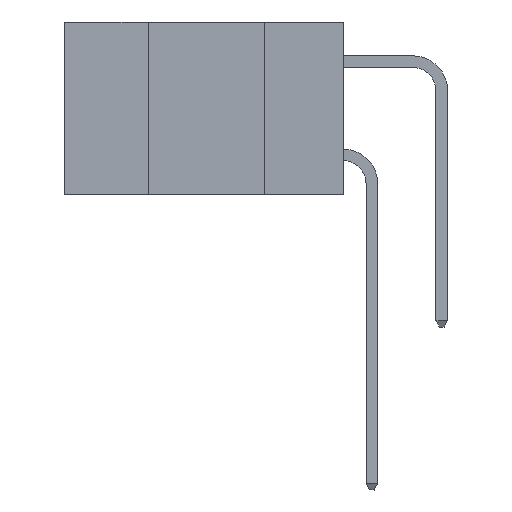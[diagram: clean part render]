
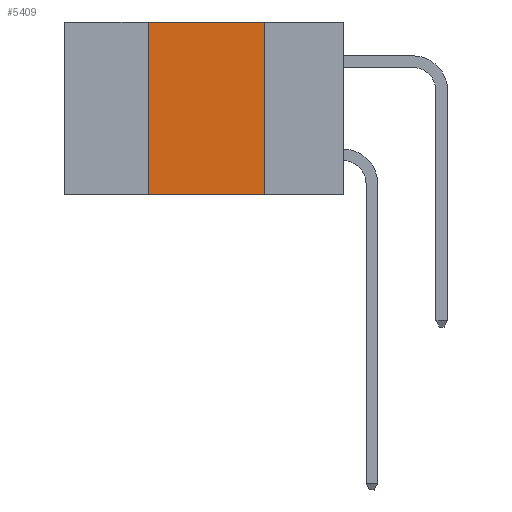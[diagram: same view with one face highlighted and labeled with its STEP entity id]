
A CAD part, left-side view. The second image highlights one B-rep face of the part: STEP entity #5409.
In plain terms, the highlighted planar face has unit normal (-1, 0, 0).
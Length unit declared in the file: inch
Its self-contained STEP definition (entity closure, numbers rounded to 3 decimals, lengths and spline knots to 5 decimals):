
#518 = LINE ( 'NONE', #1410, #14689 ) ;
#894 = VERTEX_POINT ( 'NONE', #16737 ) ;
#1314 = ORIENTED_EDGE ( 'NONE', *, *, #8282, .F. ) ;
#1405 = LINE ( 'NONE', #14857, #15516 ) ;
#1410 = CARTESIAN_POINT ( 'NONE',  ( 0., 0.6, 0. ) ) ;
#2144 = VECTOR ( 'NONE', #6854, 39.37008 ) ;
#2225 = VERTEX_POINT ( 'NONE', #10074 ) ;
#2368 = CARTESIAN_POINT ( 'NONE',  ( 0., 0.42, 0. ) ) ;
#2637 = DIRECTION ( 'NONE',  ( 0., -1., 0. ) ) ;
#4233 = FACE_OUTER_BOUND ( 'NONE', #9931, .T. ) ;
#4926 = CARTESIAN_POINT ( 'NONE',  ( 0., 0.6, 0. ) ) ;
#5344 = LINE ( 'NONE', #15822, #12545 ) ;
#5409 = ADVANCED_FACE ( 'NONE', ( #4233 ), #13362, .F. ) ;
#5485 = CARTESIAN_POINT ( 'NONE',  ( 0., 0.42, 0. ) ) ;
#5581 = DIRECTION ( 'NONE',  ( 0., -1., 0. ) ) ;
#6372 = DIRECTION ( 'NONE',  ( 0., 0., -1. ) ) ;
#6854 = DIRECTION ( 'NONE',  ( 0., 0., 1. ) ) ;
#7227 = VERTEX_POINT ( 'NONE', #8674 ) ;
#8282 = EDGE_CURVE ( 'NONE', #7227, #15948, #16612, .T. ) ;
#8403 = ORIENTED_EDGE ( 'NONE', *, *, #9039, .F. ) ;
#8674 = CARTESIAN_POINT ( 'NONE',  ( 0., 0.42, -0.37 ) ) ;
#9039 = EDGE_CURVE ( 'NONE', #15948, #894, #518, .T. ) ;
#9414 = DIRECTION ( 'NONE',  ( 0., 0., -1. ) ) ;
#9931 = EDGE_LOOP ( 'NONE', ( #14803, #8403, #1314, #10941 ) ) ;
#10074 = CARTESIAN_POINT ( 'NONE',  ( 0., 0.17, -0.37 ) ) ;
#10941 = ORIENTED_EDGE ( 'NONE', *, *, #17530, .T. ) ;
#12545 = VECTOR ( 'NONE', #6372, 39.37008 ) ;
#13362 = PLANE ( 'NONE',  #13819 ) ;
#13819 = AXIS2_PLACEMENT_3D ( 'NONE', #4926, #14558, #9414 ) ;
#14558 = DIRECTION ( 'NONE',  ( 1., 0., 0. ) ) ;
#14689 = VECTOR ( 'NONE', #5581, 39.37008 ) ;
#14803 = ORIENTED_EDGE ( 'NONE', *, *, #16465, .F. ) ;
#14857 = CARTESIAN_POINT ( 'NONE',  ( 0., 0.6, -0.37 ) ) ;
#15516 = VECTOR ( 'NONE', #2637, 39.37008 ) ;
#15822 = CARTESIAN_POINT ( 'NONE',  ( 0., 0.17, 0. ) ) ;
#15948 = VERTEX_POINT ( 'NONE', #2368 ) ;
#16465 = EDGE_CURVE ( 'NONE', #894, #2225, #5344, .T. ) ;
#16612 = LINE ( 'NONE', #5485, #2144 ) ;
#16737 = CARTESIAN_POINT ( 'NONE',  ( 0., 0.17, 0. ) ) ;
#17530 = EDGE_CURVE ( 'NONE', #7227, #2225, #1405, .T. ) ;
